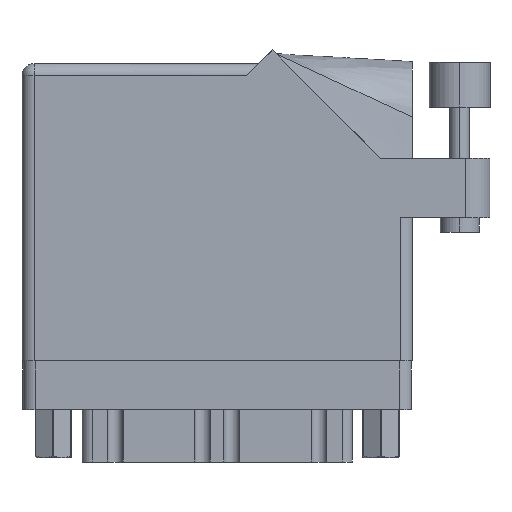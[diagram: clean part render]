
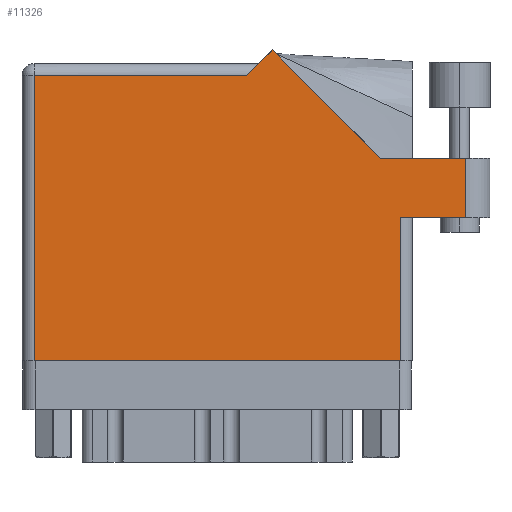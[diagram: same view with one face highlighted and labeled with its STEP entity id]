
A CAD part, front view. The second image highlights one B-rep face of the part: STEP entity #11326.
In plain terms, the highlighted face is planar.
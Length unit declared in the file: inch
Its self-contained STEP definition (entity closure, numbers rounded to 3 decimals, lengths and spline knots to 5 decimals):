
#379 = ORIENTED_EDGE ( 'NONE', *, *, #18883, .T. ) ;
#1360 = VERTEX_POINT ( 'NONE', #46210 ) ;
#1849 = EDGE_CURVE ( 'NONE', #42374, #3790, #24296, .T. ) ;
#1927 = DIRECTION ( 'NONE',  ( -0.707, -0.707, 0. ) ) ;
#3790 = VERTEX_POINT ( 'NONE', #32422 ) ;
#4758 = ORIENTED_EDGE ( 'NONE', *, *, #44042, .T. ) ;
#4989 = EDGE_LOOP ( 'NONE', ( #41853, #9201, #33038, #7402, #40651, #4758, #23421, #379, #9680 ) ) ;
#5340 = CARTESIAN_POINT ( 'NONE',  ( 0.062, 1.468, 0. ) ) ;
#5613 = VECTOR ( 'NONE', #38814, 39.37008 ) ;
#6310 = VECTOR ( 'NONE', #33583, 39.37008 ) ;
#7402 = ORIENTED_EDGE ( 'NONE', *, *, #1849, .T. ) ;
#9080 = FACE_OUTER_BOUND ( 'NONE', #4989, .T. ) ;
#9201 = ORIENTED_EDGE ( 'NONE', *, *, #27207, .T. ) ;
#9310 = LINE ( 'NONE', #24181, #5613 ) ;
#9680 = ORIENTED_EDGE ( 'NONE', *, *, #15652, .T. ) ;
#10120 = CARTESIAN_POINT ( 'NONE',  ( 1.948, 0., 0. ) ) ;
#10154 = VERTEX_POINT ( 'NONE', #36635 ) ;
#11326 = ADVANCED_FACE ( 'NONE', ( #9080 ), #23709, .F. ) ;
#11906 = CARTESIAN_POINT ( 'NONE',  ( 2.285, 1.044, 0. ) ) ;
#12018 = DIRECTION ( 'NONE',  ( 0., 1., 0. ) ) ;
#12267 = VECTOR ( 'NONE', #46719, 39.37008 ) ;
#12391 = VERTEX_POINT ( 'NONE', #33297 ) ;
#14416 = VECTOR ( 'NONE', #45895, 39.37008 ) ;
#14887 = AXIS2_PLACEMENT_3D ( 'NONE', #30441, #34282, #27092 ) ;
#15138 = DIRECTION ( 'NONE',  ( 1., 0., 0. ) ) ;
#15652 = EDGE_CURVE ( 'NONE', #41936, #19551, #22104, .T. ) ;
#16020 = LINE ( 'NONE', #20337, #22424 ) ;
#16279 = CARTESIAN_POINT ( 'NONE',  ( 0.062, 0., 0. ) ) ;
#17148 = VECTOR ( 'NONE', #12018, 39.37008 ) ;
#18883 = EDGE_CURVE ( 'NONE', #43269, #41936, #44172, .T. ) ;
#19551 = VERTEX_POINT ( 'NONE', #38104 ) ;
#20106 = DIRECTION ( 'NONE',  ( 1., 0., 0. ) ) ;
#20337 = CARTESIAN_POINT ( 'NONE',  ( 2.01, 0.737, 0. ) ) ;
#20394 = LINE ( 'NONE', #38392, #20680 ) ;
#20680 = VECTOR ( 'NONE', #1927, 39.37008 ) ;
#21179 = CARTESIAN_POINT ( 'NONE',  ( 1.84442, 1.044, 0. ) ) ;
#22104 = LINE ( 'NONE', #33601, #17148 ) ;
#22424 = VECTOR ( 'NONE', #20106, 39.37008 ) ;
#23421 = ORIENTED_EDGE ( 'NONE', *, *, #37528, .T. ) ;
#23505 = CARTESIAN_POINT ( 'NONE',  ( 0., 1.468, 0. ) ) ;
#23709 = PLANE ( 'NONE',  #14887 ) ;
#24181 = CARTESIAN_POINT ( 'NONE',  ( 0.062, 0., 0. ) ) ;
#24296 = LINE ( 'NONE', #21179, #14416 ) ;
#26149 = VECTOR ( 'NONE', #26524, 39.37008 ) ;
#26524 = DIRECTION ( 'NONE',  ( 0., 1., 0. ) ) ;
#27092 = DIRECTION ( 'NONE',  ( -1., 0., 0. ) ) ;
#27207 = EDGE_CURVE ( 'NONE', #1360, #10154, #30370, .T. ) ;
#30088 = VERTEX_POINT ( 'NONE', #5340 ) ;
#30370 = LINE ( 'NONE', #11906, #26149 ) ;
#30441 = CARTESIAN_POINT ( 'NONE',  ( 0., 1.53, 0. ) ) ;
#32084 = CARTESIAN_POINT ( 'NONE',  ( 2.41, 1.044, 0. ) ) ;
#32422 = CARTESIAN_POINT ( 'NONE',  ( 1.28771, 1.60071, 0. ) ) ;
#32450 = CARTESIAN_POINT ( 'NONE',  ( 1.84442, 1.044, 0. ) ) ;
#33038 = ORIENTED_EDGE ( 'NONE', *, *, #34110, .T. ) ;
#33297 = CARTESIAN_POINT ( 'NONE',  ( 1.155, 1.468, 0. ) ) ;
#33583 = DIRECTION ( 'NONE',  ( -1., 0., 0. ) ) ;
#33601 = CARTESIAN_POINT ( 'NONE',  ( 1.948, 0.737, 0. ) ) ;
#33710 = VECTOR ( 'NONE', #15138, 39.37008 ) ;
#33924 = EDGE_CURVE ( 'NONE', #3790, #12391, #20394, .T. ) ;
#34110 = EDGE_CURVE ( 'NONE', #10154, #42374, #42649, .T. ) ;
#34282 = DIRECTION ( 'NONE',  ( 0., 0., -1. ) ) ;
#36635 = CARTESIAN_POINT ( 'NONE',  ( 2.285, 1.044, 0. ) ) ;
#37528 = EDGE_CURVE ( 'NONE', #30088, #43269, #9310, .T. ) ;
#38104 = CARTESIAN_POINT ( 'NONE',  ( 1.948, 0.737, 0. ) ) ;
#38392 = CARTESIAN_POINT ( 'NONE',  ( 1.217, 1.53, 0. ) ) ;
#38669 = EDGE_CURVE ( 'NONE', #19551, #1360, #16020, .T. ) ;
#38814 = DIRECTION ( 'NONE',  ( 0., -1., 0. ) ) ;
#40651 = ORIENTED_EDGE ( 'NONE', *, *, #33924, .T. ) ;
#40802 = LINE ( 'NONE', #23505, #6310 ) ;
#40822 = CARTESIAN_POINT ( 'NONE',  ( 0., 0., 0. ) ) ;
#41853 = ORIENTED_EDGE ( 'NONE', *, *, #38669, .T. ) ;
#41936 = VERTEX_POINT ( 'NONE', #10120 ) ;
#42374 = VERTEX_POINT ( 'NONE', #32450 ) ;
#42649 = LINE ( 'NONE', #32084, #12267 ) ;
#43269 = VERTEX_POINT ( 'NONE', #16279 ) ;
#44042 = EDGE_CURVE ( 'NONE', #12391, #30088, #40802, .T. ) ;
#44172 = LINE ( 'NONE', #40822, #33710 ) ;
#45895 = DIRECTION ( 'NONE',  ( -0.707, 0.707, 0. ) ) ;
#46210 = CARTESIAN_POINT ( 'NONE',  ( 2.285, 0.737, 0. ) ) ;
#46719 = DIRECTION ( 'NONE',  ( -1., 0., 0. ) ) ;
